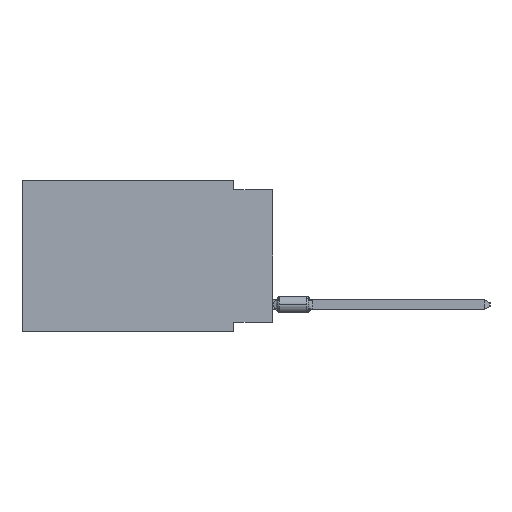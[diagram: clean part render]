
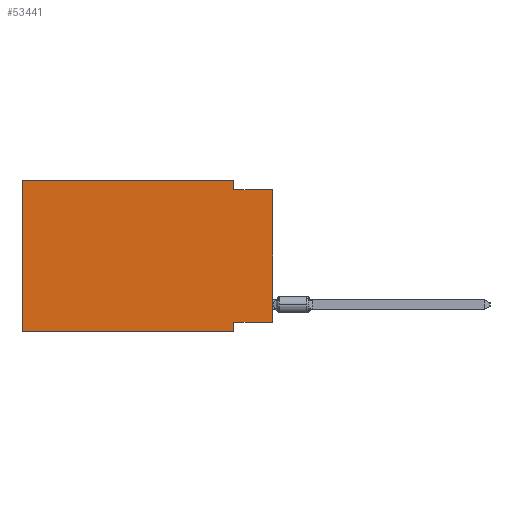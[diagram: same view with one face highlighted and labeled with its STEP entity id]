
A CAD part, left-side view. The second image highlights one B-rep face of the part: STEP entity #53441.
In plain terms, the highlighted planar face has unit normal (-1, 0, 0).
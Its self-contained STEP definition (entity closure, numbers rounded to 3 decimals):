
#33 = ORIENTED_EDGE ( 'NONE', *, *, #17669, .F. ) ;
#532 = ORIENTED_EDGE ( 'NONE', *, *, #57605, .T. ) ;
#746 = VERTEX_POINT ( 'NONE', #17543 ) ;
#905 = ORIENTED_EDGE ( 'NONE', *, *, #10962, .F. ) ;
#1003 = CARTESIAN_POINT ( 'NONE',  ( 0., 0., 0. ) ) ;
#1431 = ORIENTED_EDGE ( 'NONE', *, *, #49831, .F. ) ;
#2138 = VERTEX_POINT ( 'NONE', #13647 ) ;
#5445 = CARTESIAN_POINT ( 'NONE',  ( 0., 16.383, 0. ) ) ;
#5493 = LINE ( 'NONE', #1003, #46447 ) ;
#7484 = DIRECTION ( 'NONE',  ( 0., 0., -1. ) ) ;
#10962 = EDGE_CURVE ( 'NONE', #16204, #2138, #17202, .T. ) ;
#13647 = CARTESIAN_POINT ( 'NONE',  ( 0., 0., -0.635 ) ) ;
#15155 = EDGE_CURVE ( 'NONE', #17851, #2138, #5493, .T. ) ;
#16204 = VERTEX_POINT ( 'NONE', #56560 ) ;
#16351 = VERTEX_POINT ( 'NONE', #25318 ) ;
#17202 = LINE ( 'NONE', #35509, #42798 ) ;
#17543 = CARTESIAN_POINT ( 'NONE',  ( 0., 2.54, -9.271 ) ) ;
#17669 = EDGE_CURVE ( 'NONE', #746, #52155, #58124, .T. ) ;
#17851 = VERTEX_POINT ( 'NONE', #25459 ) ;
#17862 = LINE ( 'NONE', #58729, #51303 ) ;
#18044 = FACE_OUTER_BOUND ( 'NONE', #42453, .T. ) ;
#18761 = DIRECTION ( 'NONE',  ( 0., 1., 0. ) ) ;
#18935 = DIRECTION ( 'NONE',  ( 1., 0., 0. ) ) ;
#18951 = LINE ( 'NONE', #19547, #43361 ) ;
#19547 = CARTESIAN_POINT ( 'NONE',  ( 0., 16.383, 0. ) ) ;
#19932 = VECTOR ( 'NONE', #7484, 1000. ) ;
#21759 = DIRECTION ( 'NONE',  ( 0., 0., -1. ) ) ;
#22498 = VERTEX_POINT ( 'NONE', #54719 ) ;
#23204 = ORIENTED_EDGE ( 'NONE', *, *, #58926, .F. ) ;
#23744 = DIRECTION ( 'NONE',  ( 0., -1., 0. ) ) ;
#25318 = CARTESIAN_POINT ( 'NONE',  ( 0., 16.383, 0. ) ) ;
#25459 = CARTESIAN_POINT ( 'NONE',  ( 0., 0., -9.271 ) ) ;
#29798 = ORIENTED_EDGE ( 'NONE', *, *, #34399, .F. ) ;
#31303 = VECTOR ( 'NONE', #21759, 1000. ) ;
#32443 = ORIENTED_EDGE ( 'NONE', *, *, #42058, .F. ) ;
#33372 = DIRECTION ( 'NONE',  ( 0., 0., 1. ) ) ;
#33493 = CARTESIAN_POINT ( 'NONE',  ( 0., 2.54, -9.906 ) ) ;
#33888 = CARTESIAN_POINT ( 'NONE',  ( 0., 16.383, 0. ) ) ;
#34399 = EDGE_CURVE ( 'NONE', #22498, #16204, #39581, .T. ) ;
#34992 = CARTESIAN_POINT ( 'NONE',  ( 0., 2.54, -9.906 ) ) ;
#35509 = CARTESIAN_POINT ( 'NONE',  ( 0., 0., -0.635 ) ) ;
#35594 = AXIS2_PLACEMENT_3D ( 'NONE', #5445, #18935, #55577 ) ;
#35887 = CARTESIAN_POINT ( 'NONE',  ( 0., 0., -9.271 ) ) ;
#36448 = DIRECTION ( 'NONE',  ( 0., -1., 0. ) ) ;
#38371 = VECTOR ( 'NONE', #52219, 1000. ) ;
#39581 = LINE ( 'NONE', #48599, #19932 ) ;
#40381 = LINE ( 'NONE', #35887, #52331 ) ;
#42058 = EDGE_CURVE ( 'NONE', #53796, #16351, #57309, .T. ) ;
#42453 = EDGE_LOOP ( 'NONE', ( #53511, #905, #29798, #1431, #32443, #532, #33, #23204 ) ) ;
#42798 = VECTOR ( 'NONE', #53851, 1000. ) ;
#43361 = VECTOR ( 'NONE', #23744, 1000. ) ;
#46190 = CARTESIAN_POINT ( 'NONE',  ( 0., 16.383, -9.906 ) ) ;
#46447 = VECTOR ( 'NONE', #33372, 1000. ) ;
#46560 = PLANE ( 'NONE',  #35594 ) ;
#48599 = CARTESIAN_POINT ( 'NONE',  ( 0., 2.54, 0. ) ) ;
#49831 = EDGE_CURVE ( 'NONE', #16351, #22498, #18951, .T. ) ;
#51303 = VECTOR ( 'NONE', #36448, 1000. ) ;
#52155 = VERTEX_POINT ( 'NONE', #33493 ) ;
#52219 = DIRECTION ( 'NONE',  ( 0., 0., 1. ) ) ;
#52331 = VECTOR ( 'NONE', #18761, 1000. ) ;
#53441 = ADVANCED_FACE ( 'NONE', ( #18044 ), #46560, .F. ) ;
#53511 = ORIENTED_EDGE ( 'NONE', *, *, #15155, .T. ) ;
#53796 = VERTEX_POINT ( 'NONE', #46190 ) ;
#53851 = DIRECTION ( 'NONE',  ( 0., -1., 0. ) ) ;
#54719 = CARTESIAN_POINT ( 'NONE',  ( 0., 2.54, 0. ) ) ;
#55577 = DIRECTION ( 'NONE',  ( 0., 0., -1. ) ) ;
#56560 = CARTESIAN_POINT ( 'NONE',  ( 0., 2.54, -0.635 ) ) ;
#57309 = LINE ( 'NONE', #33888, #38371 ) ;
#57605 = EDGE_CURVE ( 'NONE', #53796, #52155, #17862, .T. ) ;
#58124 = LINE ( 'NONE', #34992, #31303 ) ;
#58729 = CARTESIAN_POINT ( 'NONE',  ( 0., 16.383, -9.906 ) ) ;
#58926 = EDGE_CURVE ( 'NONE', #17851, #746, #40381, .T. ) ;
